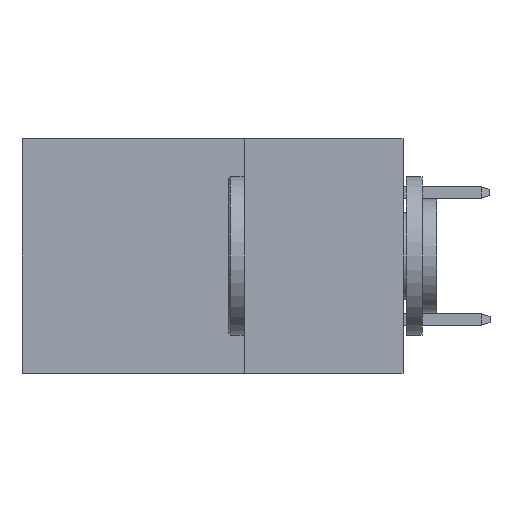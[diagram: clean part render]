
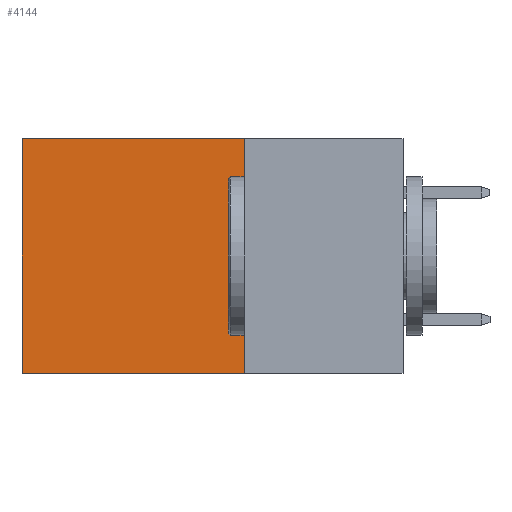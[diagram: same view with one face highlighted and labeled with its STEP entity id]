
A CAD part, left-side view. The second image highlights one B-rep face of the part: STEP entity #4144.
In plain terms, the highlighted planar face has unit normal (-1, 0, 0).
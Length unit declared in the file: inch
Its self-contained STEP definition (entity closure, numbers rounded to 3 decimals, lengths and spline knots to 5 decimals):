
#24 = VECTOR ( 'NONE', #2161, 39.37008 ) ;
#46 = VERTEX_POINT ( 'NONE', #1049 ) ;
#131 = VERTEX_POINT ( 'NONE', #5051 ) ;
#198 = ORIENTED_EDGE ( 'NONE', *, *, #6805, .T. ) ;
#238 = EDGE_CURVE ( 'NONE', #46, #131, #2201, .T. ) ;
#765 = LINE ( 'NONE', #3744, #5895 ) ;
#1049 = CARTESIAN_POINT ( 'NONE',  ( 0.2875, 0.25, 0. ) ) ;
#1137 = EDGE_CURVE ( 'NONE', #46, #6131, #9022, .T. ) ;
#1289 = ORIENTED_EDGE ( 'NONE', *, *, #4099, .F. ) ;
#1576 = EDGE_LOOP ( 'NONE', ( #198, #1289, #7947, #7223 ) ) ;
#1934 = VECTOR ( 'NONE', #8179, 39.37008 ) ;
#2161 = DIRECTION ( 'NONE',  ( 0., 0., -1. ) ) ;
#2201 = LINE ( 'NONE', #5193, #1934 ) ;
#2532 = DIRECTION ( 'NONE',  ( 0., 0., -1. ) ) ;
#3006 = DIRECTION ( 'NONE',  ( 0., 1., 0. ) ) ;
#3744 = CARTESIAN_POINT ( 'NONE',  ( 0.2875, 0.25, -0.37 ) ) ;
#4099 = EDGE_CURVE ( 'NONE', #6131, #6832, #765, .T. ) ;
#4144 = ADVANCED_FACE ( 'NONE', ( #4826 ), #5605, .F. ) ;
#4734 = DIRECTION ( 'NONE',  ( 0., 0., -1. ) ) ;
#4826 = FACE_OUTER_BOUND ( 'NONE', #1576, .T. ) ;
#4909 = VECTOR ( 'NONE', #2532, 39.37008 ) ;
#5051 = CARTESIAN_POINT ( 'NONE',  ( 0.2875, 0.6, 0. ) ) ;
#5193 = CARTESIAN_POINT ( 'NONE',  ( 0.2875, 0.25, 0. ) ) ;
#5422 = CARTESIAN_POINT ( 'NONE',  ( 0.2875, 0.6, 0. ) ) ;
#5430 = AXIS2_PLACEMENT_3D ( 'NONE', #5460, #5561, #4734 ) ;
#5460 = CARTESIAN_POINT ( 'NONE',  ( 0.2875, 0.25, 0. ) ) ;
#5561 = DIRECTION ( 'NONE',  ( 1., 0., 0. ) ) ;
#5605 = PLANE ( 'NONE',  #5430 ) ;
#5895 = VECTOR ( 'NONE', #3006, 39.37008 ) ;
#6131 = VERTEX_POINT ( 'NONE', #8784 ) ;
#6805 = EDGE_CURVE ( 'NONE', #131, #6832, #9138, .T. ) ;
#6832 = VERTEX_POINT ( 'NONE', #6929 ) ;
#6929 = CARTESIAN_POINT ( 'NONE',  ( 0.2875, 0.6, -0.37 ) ) ;
#7223 = ORIENTED_EDGE ( 'NONE', *, *, #238, .T. ) ;
#7947 = ORIENTED_EDGE ( 'NONE', *, *, #1137, .F. ) ;
#8179 = DIRECTION ( 'NONE',  ( 0., 1., 0. ) ) ;
#8784 = CARTESIAN_POINT ( 'NONE',  ( 0.2875, 0.25, -0.37 ) ) ;
#9022 = LINE ( 'NONE', #9647, #24 ) ;
#9138 = LINE ( 'NONE', #5422, #4909 ) ;
#9647 = CARTESIAN_POINT ( 'NONE',  ( 0.2875, 0.25, 0. ) ) ;
